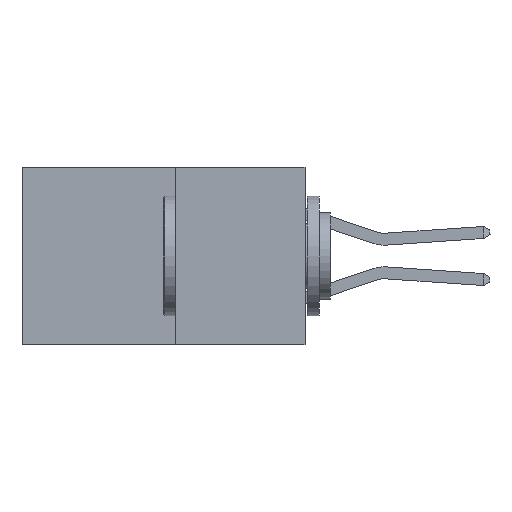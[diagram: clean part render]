
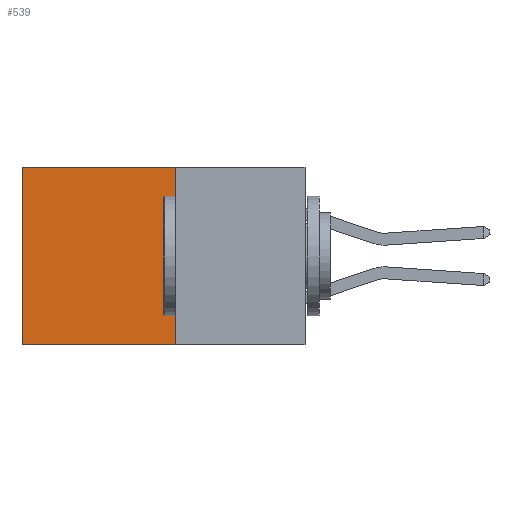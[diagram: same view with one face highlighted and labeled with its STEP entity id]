
A CAD part, left-side view. The second image highlights one B-rep face of the part: STEP entity #539.
In plain terms, the highlighted planar face has unit normal (-1, 0, 0).
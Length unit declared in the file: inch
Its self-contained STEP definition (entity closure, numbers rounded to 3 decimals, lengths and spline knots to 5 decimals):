
#270 = AXIS2_PLACEMENT_3D ( 'NONE', #2683, #5413, #3791 ) ;
#460 = VERTEX_POINT ( 'NONE', #5121 ) ;
#539 = ADVANCED_FACE ( 'NONE', ( #2553 ), #5742, .F. ) ;
#984 = LINE ( 'NONE', #7848, #7873 ) ;
#1259 = EDGE_CURVE ( 'NONE', #6704, #9017, #9092, .T. ) ;
#1288 = EDGE_CURVE ( 'NONE', #6704, #460, #7414, .T. ) ;
#1595 = LINE ( 'NONE', #8399, #3313 ) ;
#2553 = FACE_OUTER_BOUND ( 'NONE', #4138, .T. ) ;
#2572 = DIRECTION ( 'NONE',  ( 0., 0., -1. ) ) ;
#2683 = CARTESIAN_POINT ( 'NONE',  ( 0.277, 0.27, -0.37 ) ) ;
#2827 = CARTESIAN_POINT ( 'NONE',  ( 0.277, 0.27, 0. ) ) ;
#2974 = DIRECTION ( 'NONE',  ( 0., 1., 0. ) ) ;
#3002 = CARTESIAN_POINT ( 'NONE',  ( 0.277, 0.27, 0. ) ) ;
#3313 = VECTOR ( 'NONE', #5037, 39.37008 ) ;
#3444 = VECTOR ( 'NONE', #2572, 39.37008 ) ;
#3566 = EDGE_CURVE ( 'NONE', #460, #5033, #984, .T. ) ;
#3791 = DIRECTION ( 'NONE',  ( 0., 0., -1. ) ) ;
#3929 = VECTOR ( 'NONE', #2974, 39.37008 ) ;
#4138 = EDGE_LOOP ( 'NONE', ( #7413, #7393, #7364, #7162 ) ) ;
#4971 = CARTESIAN_POINT ( 'NONE',  ( 0.277, 0.27, -0.37 ) ) ;
#5033 = VERTEX_POINT ( 'NONE', #7983 ) ;
#5037 = DIRECTION ( 'NONE',  ( 0., 0., -1. ) ) ;
#5121 = CARTESIAN_POINT ( 'NONE',  ( 0.277, 0.27, -0.37 ) ) ;
#5413 = DIRECTION ( 'NONE',  ( 1., 0., 0. ) ) ;
#5742 = PLANE ( 'NONE',  #270 ) ;
#6704 = VERTEX_POINT ( 'NONE', #3002 ) ;
#7162 = ORIENTED_EDGE ( 'NONE', *, *, #1259, .T. ) ;
#7364 = ORIENTED_EDGE ( 'NONE', *, *, #1288, .F. ) ;
#7393 = ORIENTED_EDGE ( 'NONE', *, *, #3566, .F. ) ;
#7413 = ORIENTED_EDGE ( 'NONE', *, *, #8642, .T. ) ;
#7414 = LINE ( 'NONE', #4971, #3444 ) ;
#7848 = CARTESIAN_POINT ( 'NONE',  ( 0.277, 0.27, -0.37 ) ) ;
#7873 = VECTOR ( 'NONE', #8729, 39.37008 ) ;
#7983 = CARTESIAN_POINT ( 'NONE',  ( 0.277, 0.59, -0.37 ) ) ;
#8110 = CARTESIAN_POINT ( 'NONE',  ( 0.277, 0.59, 0. ) ) ;
#8399 = CARTESIAN_POINT ( 'NONE',  ( 0.277, 0.59, -0.37 ) ) ;
#8642 = EDGE_CURVE ( 'NONE', #9017, #5033, #1595, .T. ) ;
#8729 = DIRECTION ( 'NONE',  ( 0., 1., 0. ) ) ;
#9017 = VERTEX_POINT ( 'NONE', #8110 ) ;
#9092 = LINE ( 'NONE', #2827, #3929 ) ;
